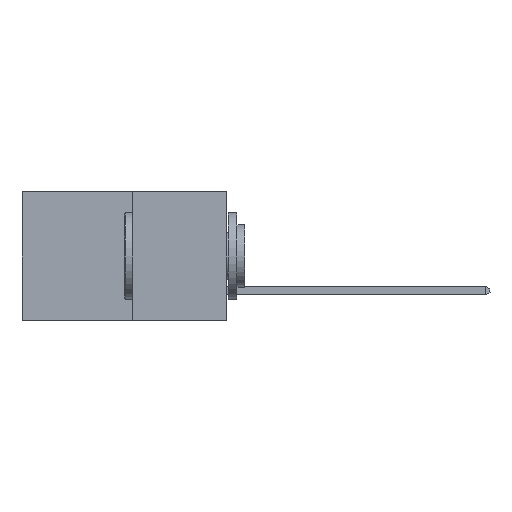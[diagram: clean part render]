
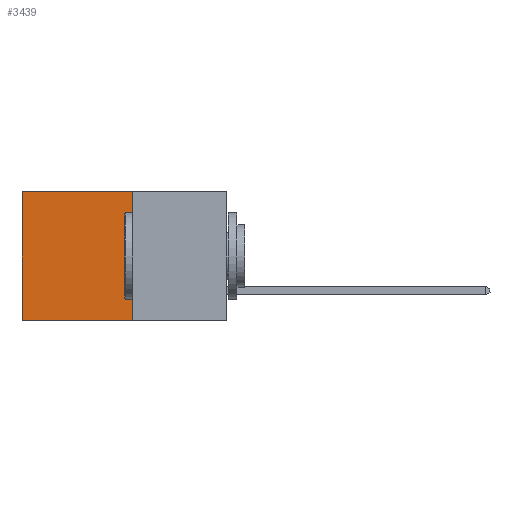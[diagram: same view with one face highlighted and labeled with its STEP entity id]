
A CAD part, left-side view. The second image highlights one B-rep face of the part: STEP entity #3439.
In plain terms, the highlighted planar face has unit normal (-1, 0, 0).
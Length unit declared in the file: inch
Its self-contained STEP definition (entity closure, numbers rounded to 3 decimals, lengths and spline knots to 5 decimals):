
#1236 = EDGE_CURVE ( 'NONE', #4281, #2547, #1787, .T. ) ;
#1787 = LINE ( 'NONE', #12766, #4528 ) ;
#1792 = ORIENTED_EDGE ( 'NONE', *, *, #7164, .T. ) ;
#1808 = LINE ( 'NONE', #11062, #4548 ) ;
#2328 = CARTESIAN_POINT ( 'NONE',  ( 0.277, 0.59, 0. ) ) ;
#2547 = VERTEX_POINT ( 'NONE', #12808 ) ;
#2852 = VERTEX_POINT ( 'NONE', #2328 ) ;
#3127 = AXIS2_PLACEMENT_3D ( 'NONE', #13493, #13424, #13422 ) ;
#3439 = ADVANCED_FACE ( 'NONE', ( #5950 ), #13854, .F. ) ;
#3778 = CARTESIAN_POINT ( 'NONE',  ( 0.277, 0.27, -0.37 ) ) ;
#4281 = VERTEX_POINT ( 'NONE', #3778 ) ;
#4528 = VECTOR ( 'NONE', #12929, 39.37008 ) ;
#4548 = VECTOR ( 'NONE', #12258, 39.37008 ) ;
#4923 = ORIENTED_EDGE ( 'NONE', *, *, #6359, .T. ) ;
#4952 = ORIENTED_EDGE ( 'NONE', *, *, #8428, .F. ) ;
#5044 = CARTESIAN_POINT ( 'NONE',  ( 0.277, 0.59, -0.37 ) ) ;
#5666 = ORIENTED_EDGE ( 'NONE', *, *, #1236, .F. ) ;
#5950 = FACE_OUTER_BOUND ( 'NONE', #14203, .T. ) ;
#6359 = EDGE_CURVE ( 'NONE', #10965, #2852, #7689, .T. ) ;
#6755 = LINE ( 'NONE', #5044, #14953 ) ;
#7164 = EDGE_CURVE ( 'NONE', #2852, #2547, #6755, .T. ) ;
#7689 = LINE ( 'NONE', #14474, #10789 ) ;
#8428 = EDGE_CURVE ( 'NONE', #10965, #4281, #1808, .T. ) ;
#8649 = DIRECTION ( 'NONE',  ( 0., 0., -1. ) ) ;
#9144 = CARTESIAN_POINT ( 'NONE',  ( 0.277, 0.27, 0. ) ) ;
#10789 = VECTOR ( 'NONE', #14554, 39.37008 ) ;
#10965 = VERTEX_POINT ( 'NONE', #9144 ) ;
#11062 = CARTESIAN_POINT ( 'NONE',  ( 0.277, 0.27, -0.37 ) ) ;
#12258 = DIRECTION ( 'NONE',  ( 0., 0., -1. ) ) ;
#12766 = CARTESIAN_POINT ( 'NONE',  ( 0.277, 0.27, -0.37 ) ) ;
#12808 = CARTESIAN_POINT ( 'NONE',  ( 0.277, 0.59, -0.37 ) ) ;
#12929 = DIRECTION ( 'NONE',  ( 0., 1., 0. ) ) ;
#13422 = DIRECTION ( 'NONE',  ( 0., 0., -1. ) ) ;
#13424 = DIRECTION ( 'NONE',  ( 1., 0., 0. ) ) ;
#13493 = CARTESIAN_POINT ( 'NONE',  ( 0.277, 0.27, -0.37 ) ) ;
#13854 = PLANE ( 'NONE',  #3127 ) ;
#14203 = EDGE_LOOP ( 'NONE', ( #1792, #5666, #4952, #4923 ) ) ;
#14474 = CARTESIAN_POINT ( 'NONE',  ( 0.277, 0.27, 0. ) ) ;
#14554 = DIRECTION ( 'NONE',  ( 0., 1., 0. ) ) ;
#14953 = VECTOR ( 'NONE', #8649, 39.37008 ) ;
